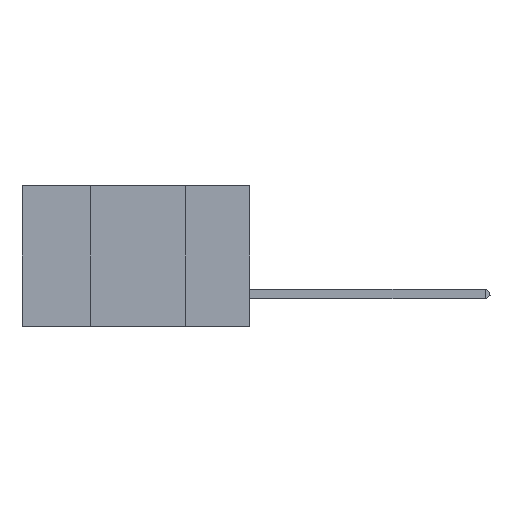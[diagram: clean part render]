
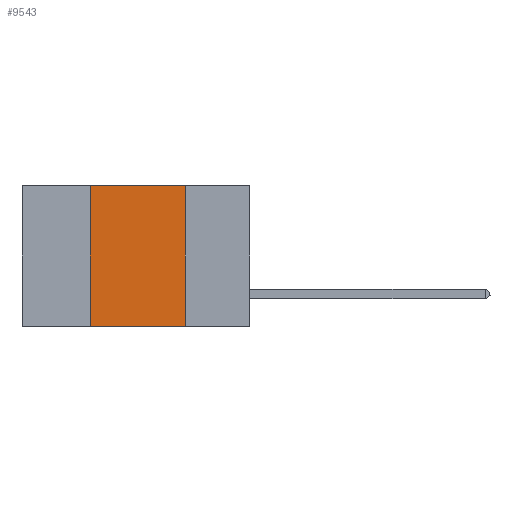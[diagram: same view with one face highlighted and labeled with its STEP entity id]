
A CAD part, left-side view. The second image highlights one B-rep face of the part: STEP entity #9543.
In plain terms, the highlighted planar face has unit normal (-1, 0, 0).
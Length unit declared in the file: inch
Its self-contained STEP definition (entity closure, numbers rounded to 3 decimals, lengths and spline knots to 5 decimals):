
#455 = CARTESIAN_POINT ( 'NONE',  ( 0., 0.6, 0. ) ) ;
#820 = ORIENTED_EDGE ( 'NONE', *, *, #10916, .F. ) ;
#1244 = CARTESIAN_POINT ( 'NONE',  ( 0., 0.17, -0.37 ) ) ;
#2006 = EDGE_CURVE ( 'NONE', #13252, #6554, #7217, .T. ) ;
#2524 = EDGE_CURVE ( 'NONE', #5322, #10722, #14545, .T. ) ;
#2598 = CARTESIAN_POINT ( 'NONE',  ( 0., 0.42, 0. ) ) ;
#2957 = PLANE ( 'NONE',  #7693 ) ;
#3250 = DIRECTION ( 'NONE',  ( 0., -1., 0. ) ) ;
#5184 = VECTOR ( 'NONE', #14895, 39.37008 ) ;
#5322 = VERTEX_POINT ( 'NONE', #16896 ) ;
#6475 = EDGE_LOOP ( 'NONE', ( #14116, #820, #14044, #16914 ) ) ;
#6554 = VERTEX_POINT ( 'NONE', #8072 ) ;
#6892 = EDGE_CURVE ( 'NONE', #13252, #10722, #7861, .T. ) ;
#7217 = LINE ( 'NONE', #2598, #13210 ) ;
#7693 = AXIS2_PLACEMENT_3D ( 'NONE', #11519, #16795, #11444 ) ;
#7861 = LINE ( 'NONE', #13272, #21388 ) ;
#8072 = CARTESIAN_POINT ( 'NONE',  ( 0., 0.42, 0. ) ) ;
#9340 = DIRECTION ( 'NONE',  ( 0., 0., 1. ) ) ;
#9543 = ADVANCED_FACE ( 'NONE', ( #16353 ), #2957, .F. ) ;
#9945 = VECTOR ( 'NONE', #21361, 39.37008 ) ;
#10722 = VERTEX_POINT ( 'NONE', #1244 ) ;
#10916 = EDGE_CURVE ( 'NONE', #6554, #5322, #21463, .T. ) ;
#11444 = DIRECTION ( 'NONE',  ( 0., 0., -1. ) ) ;
#11519 = CARTESIAN_POINT ( 'NONE',  ( 0., 0.6, 0. ) ) ;
#13210 = VECTOR ( 'NONE', #9340, 39.37008 ) ;
#13252 = VERTEX_POINT ( 'NONE', #20020 ) ;
#13272 = CARTESIAN_POINT ( 'NONE',  ( 0., 0.6, -0.37 ) ) ;
#14044 = ORIENTED_EDGE ( 'NONE', *, *, #2006, .F. ) ;
#14116 = ORIENTED_EDGE ( 'NONE', *, *, #2524, .F. ) ;
#14545 = LINE ( 'NONE', #14548, #9945 ) ;
#14548 = CARTESIAN_POINT ( 'NONE',  ( 0., 0.17, 0. ) ) ;
#14895 = DIRECTION ( 'NONE',  ( 0., -1., 0. ) ) ;
#16353 = FACE_OUTER_BOUND ( 'NONE', #6475, .T. ) ;
#16795 = DIRECTION ( 'NONE',  ( 1., 0., 0. ) ) ;
#16896 = CARTESIAN_POINT ( 'NONE',  ( 0., 0.17, 0. ) ) ;
#16914 = ORIENTED_EDGE ( 'NONE', *, *, #6892, .T. ) ;
#20020 = CARTESIAN_POINT ( 'NONE',  ( 0., 0.42, -0.37 ) ) ;
#21361 = DIRECTION ( 'NONE',  ( 0., 0., -1. ) ) ;
#21388 = VECTOR ( 'NONE', #3250, 39.37008 ) ;
#21463 = LINE ( 'NONE', #455, #5184 ) ;
